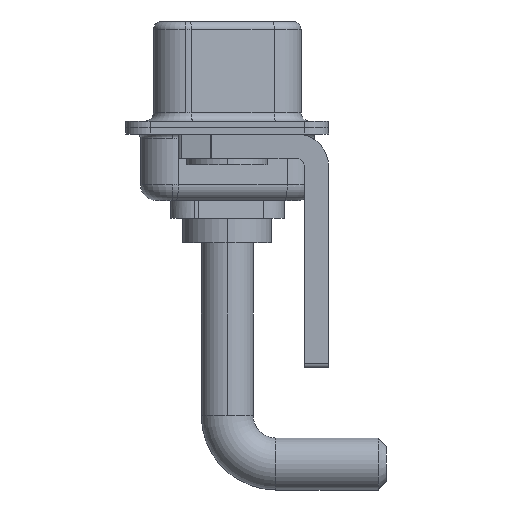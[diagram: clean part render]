
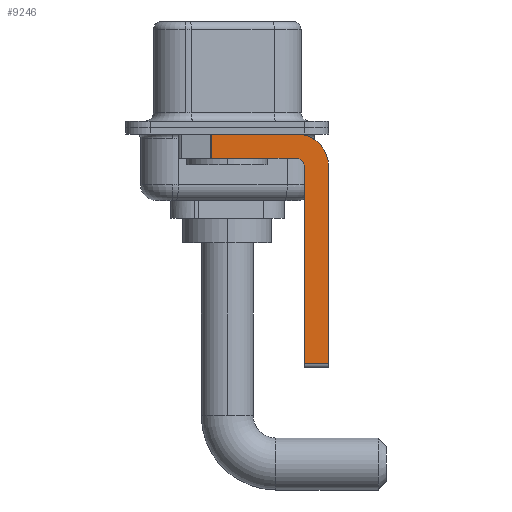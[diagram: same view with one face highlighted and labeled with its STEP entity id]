
A CAD part, left-side view. The second image highlights one B-rep face of the part: STEP entity #9246.
In plain terms, the highlighted planar face has unit normal (-1, 0, 0).
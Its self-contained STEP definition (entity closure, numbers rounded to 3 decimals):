
#141 = EDGE_CURVE ( 'NONE', #8053, #16070, #6801, .T. ) ;
#203 = DIRECTION ( 'NONE',  ( 0., 0., -1. ) ) ;
#381 = AXIS2_PLACEMENT_3D ( 'NONE', #16169, #8318, #15817 ) ;
#514 = VECTOR ( 'NONE', #203, 1000. ) ;
#668 = DIRECTION ( 'NONE',  ( 1., 0., 0. ) ) ;
#1123 = CARTESIAN_POINT ( 'NONE',  ( -2.9, -4.75, -14.8 ) ) ;
#1562 = VECTOR ( 'NONE', #13207, 1000. ) ;
#1653 = CIRCLE ( 'NONE', #7636, 0.5 ) ;
#1666 = EDGE_CURVE ( 'NONE', #16030, #3574, #9791, .T. ) ;
#1805 = VECTOR ( 'NONE', #14256, 1000. ) ;
#2142 = EDGE_CURVE ( 'NONE', #6625, #16070, #6506, .T. ) ;
#2360 = DIRECTION ( 'NONE',  ( 0., 0., 1. ) ) ;
#2477 = ORIENTED_EDGE ( 'NONE', *, *, #1666, .T. ) ;
#3233 = VECTOR ( 'NONE', #7236, 1000. ) ;
#3480 = CARTESIAN_POINT ( 'NONE',  ( -2.9, -4.25, -0.4 ) ) ;
#3537 = ORIENTED_EDGE ( 'NONE', *, *, #2142, .F. ) ;
#3574 = VERTEX_POINT ( 'NONE', #8470 ) ;
#4013 = CARTESIAN_POINT ( 'NONE',  ( -2.9, -4.75, -14.55 ) ) ;
#4134 = CARTESIAN_POINT ( 'NONE',  ( -2.9, -6.25, -2.4 ) ) ;
#4217 = EDGE_CURVE ( 'NONE', #10664, #3574, #4634, .T. ) ;
#4330 = CARTESIAN_POINT ( 'NONE',  ( -2.9, 3., -0.4 ) ) ;
#4379 = CARTESIAN_POINT ( 'NONE',  ( -2.9, 0.978, -0.4 ) ) ;
#4634 = LINE ( 'NONE', #13995, #12786 ) ;
#5280 = EDGE_CURVE ( 'NONE', #10842, #10664, #1653, .T. ) ;
#6269 = ORIENTED_EDGE ( 'NONE', *, *, #141, .T. ) ;
#6506 = LINE ( 'NONE', #4134, #514 ) ;
#6625 = VERTEX_POINT ( 'NONE', #11225 ) ;
#6801 = LINE ( 'NONE', #9098, #1562 ) ;
#6973 = CARTESIAN_POINT ( 'NONE',  ( -2.9, -4.25, -2.4 ) ) ;
#7149 = CARTESIAN_POINT ( 'NONE',  ( -2.9, 0.978, -1.9 ) ) ;
#7236 = DIRECTION ( 'NONE',  ( 0., 0., -1. ) ) ;
#7431 = DIRECTION ( 'NONE',  ( 0., 1., 0. ) ) ;
#7636 = AXIS2_PLACEMENT_3D ( 'NONE', #10353, #15459, #2360 ) ;
#8053 = VERTEX_POINT ( 'NONE', #4013 ) ;
#8318 = DIRECTION ( 'NONE',  ( 1., 0., 0. ) ) ;
#8413 = DIRECTION ( 'NONE',  ( 0., -1., 0. ) ) ;
#8425 = FACE_OUTER_BOUND ( 'NONE', #10423, .T. ) ;
#8470 = CARTESIAN_POINT ( 'NONE',  ( -2.9, 0.978, -1.9 ) ) ;
#8559 = EDGE_CURVE ( 'NONE', #15358, #6625, #14002, .T. ) ;
#8594 = CARTESIAN_POINT ( 'NONE',  ( -2.9, -4.75, -2.4 ) ) ;
#9098 = CARTESIAN_POINT ( 'NONE',  ( -2.9, -4.25, -14.55 ) ) ;
#9246 = ADVANCED_FACE ( 'NONE', ( #8425 ), #14812, .F. ) ;
#9791 = LINE ( 'NONE', #7149, #3233 ) ;
#9892 = EDGE_CURVE ( 'NONE', #8053, #10842, #15516, .T. ) ;
#10353 = CARTESIAN_POINT ( 'NONE',  ( -2.9, -4.25, -2.4 ) ) ;
#10423 = EDGE_LOOP ( 'NONE', ( #15903, #2477, #13134, #13248, #15651, #6269, #3537, #11521 ) ) ;
#10664 = VERTEX_POINT ( 'NONE', #11082 ) ;
#10842 = VERTEX_POINT ( 'NONE', #8594 ) ;
#10908 = DIRECTION ( 'NONE',  ( 0., 0., -1. ) ) ;
#11082 = CARTESIAN_POINT ( 'NONE',  ( -2.9, -4.25, -1.9 ) ) ;
#11225 = CARTESIAN_POINT ( 'NONE',  ( -2.9, -6.25, -2.4 ) ) ;
#11328 = AXIS2_PLACEMENT_3D ( 'NONE', #6973, #668, #10908 ) ;
#11521 = ORIENTED_EDGE ( 'NONE', *, *, #8559, .F. ) ;
#12477 = EDGE_CURVE ( 'NONE', #16030, #15358, #13706, .T. ) ;
#12786 = VECTOR ( 'NONE', #7431, 1000. ) ;
#13134 = ORIENTED_EDGE ( 'NONE', *, *, #4217, .F. ) ;
#13207 = DIRECTION ( 'NONE',  ( 0., -1., 0. ) ) ;
#13246 = CARTESIAN_POINT ( 'NONE',  ( -2.9, -6.25, -14.55 ) ) ;
#13248 = ORIENTED_EDGE ( 'NONE', *, *, #5280, .F. ) ;
#13706 = LINE ( 'NONE', #4330, #14767 ) ;
#13995 = CARTESIAN_POINT ( 'NONE',  ( -2.9, -4.25, -1.9 ) ) ;
#14002 = CIRCLE ( 'NONE', #381, 2. ) ;
#14256 = DIRECTION ( 'NONE',  ( 0., 0., 1. ) ) ;
#14767 = VECTOR ( 'NONE', #8413, 1000. ) ;
#14812 = PLANE ( 'NONE',  #11328 ) ;
#15358 = VERTEX_POINT ( 'NONE', #3480 ) ;
#15459 = DIRECTION ( 'NONE',  ( -1., 0., 0. ) ) ;
#15516 = LINE ( 'NONE', #1123, #1805 ) ;
#15651 = ORIENTED_EDGE ( 'NONE', *, *, #9892, .F. ) ;
#15817 = DIRECTION ( 'NONE',  ( 0., 0., -1. ) ) ;
#15903 = ORIENTED_EDGE ( 'NONE', *, *, #12477, .F. ) ;
#16030 = VERTEX_POINT ( 'NONE', #4379 ) ;
#16070 = VERTEX_POINT ( 'NONE', #13246 ) ;
#16169 = CARTESIAN_POINT ( 'NONE',  ( -2.9, -4.25, -2.4 ) ) ;
